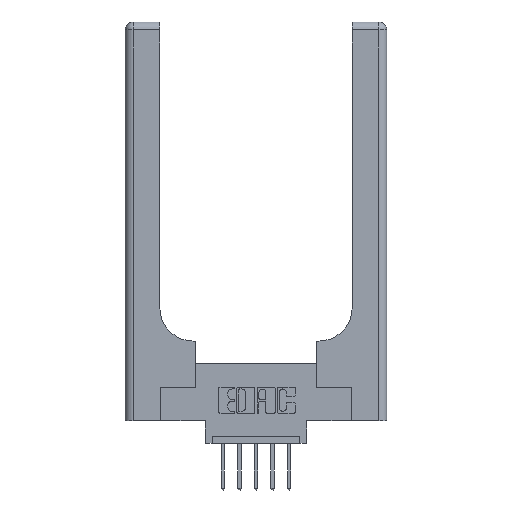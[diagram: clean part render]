
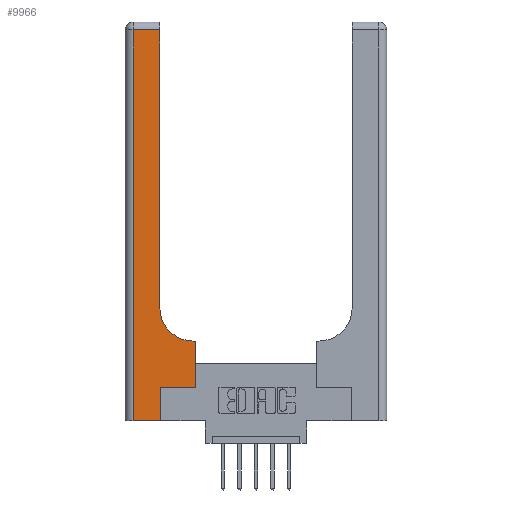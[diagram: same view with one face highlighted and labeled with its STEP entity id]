
A CAD part, top view. The second image highlights one B-rep face of the part: STEP entity #9966.
In plain terms, the highlighted planar face has unit normal (0, 0, 1).
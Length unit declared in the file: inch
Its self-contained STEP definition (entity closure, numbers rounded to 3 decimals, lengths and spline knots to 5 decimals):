
#115 = EDGE_CURVE ( 'NONE', #11340, #2435, #12974, .T. ) ;
#351 = EDGE_CURVE ( 'NONE', #13493, #11340, #6523, .T. ) ;
#663 = DIRECTION ( 'NONE',  ( 1., 0., 0. ) ) ;
#1074 = CARTESIAN_POINT ( 'NONE',  ( 0.26, 3., 0.37 ) ) ;
#1745 = ORIENTED_EDGE ( 'NONE', *, *, #12479, .T. ) ;
#1832 = VECTOR ( 'NONE', #2896, 39.37008 ) ;
#1881 = CARTESIAN_POINT ( 'NONE',  ( 0.265, 0., 0.37 ) ) ;
#1899 = CARTESIAN_POINT ( 'NONE',  ( 0.06, 0., 0.37 ) ) ;
#1978 = PLANE ( 'NONE',  #11228 ) ;
#1983 = VERTEX_POINT ( 'NONE', #2125 ) ;
#2125 = CARTESIAN_POINT ( 'NONE',  ( 0.265, 0.25, 0.37 ) ) ;
#2240 = LINE ( 'NONE', #9895, #9949 ) ;
#2265 = DIRECTION ( 'NONE',  ( 0., 1., 0. ) ) ;
#2435 = VERTEX_POINT ( 'NONE', #8600 ) ;
#2511 = LINE ( 'NONE', #13506, #4847 ) ;
#2845 = ORIENTED_EDGE ( 'NONE', *, *, #7144, .T. ) ;
#2877 = CARTESIAN_POINT ( 'NONE',  ( 0., 0., 0.37 ) ) ;
#2896 = DIRECTION ( 'NONE',  ( 1., 0., 0. ) ) ;
#2944 = DIRECTION ( 'NONE',  ( 1., 0., 0. ) ) ;
#3007 = CARTESIAN_POINT ( 'NONE',  ( 0.528, 0.25, 0.37 ) ) ;
#3360 = DIRECTION ( 'NONE',  ( -1., 0., 0. ) ) ;
#3731 = CARTESIAN_POINT ( 'NONE',  ( 0.51, 0.6, 0.37 ) ) ;
#3984 = ORIENTED_EDGE ( 'NONE', *, *, #6684, .T. ) ;
#4398 = CARTESIAN_POINT ( 'NONE',  ( 0.26, 0.6, 0.37 ) ) ;
#4427 = DIRECTION ( 'NONE',  ( 0., 1., 0. ) ) ;
#4812 = CARTESIAN_POINT ( 'NONE',  ( 0.528, 0.6, 0.37 ) ) ;
#4847 = VECTOR ( 'NONE', #4970, 39.37008 ) ;
#4906 = VERTEX_POINT ( 'NONE', #11835 ) ;
#4970 = DIRECTION ( 'NONE',  ( 0., -1., 0. ) ) ;
#5153 = CARTESIAN_POINT ( 'NONE',  ( 0.51, 0.85, 0.37 ) ) ;
#5369 = LINE ( 'NONE', #1074, #9426 ) ;
#5440 = DIRECTION ( 'NONE',  ( -1., 0., 0. ) ) ;
#5684 = EDGE_CURVE ( 'NONE', #6276, #6984, #13389, .T. ) ;
#5814 = VECTOR ( 'NONE', #11286, 39.37008 ) ;
#6146 = VECTOR ( 'NONE', #2944, 39.37008 ) ;
#6276 = VERTEX_POINT ( 'NONE', #1899 ) ;
#6316 = ORIENTED_EDGE ( 'NONE', *, *, #13641, .T. ) ;
#6484 = LINE ( 'NONE', #11822, #7961 ) ;
#6523 = LINE ( 'NONE', #4398, #5814 ) ;
#6579 = ORIENTED_EDGE ( 'NONE', *, *, #115, .T. ) ;
#6678 = ORIENTED_EDGE ( 'NONE', *, *, #351, .T. ) ;
#6684 = EDGE_CURVE ( 'NONE', #11587, #13493, #6484, .T. ) ;
#6935 = AXIS2_PLACEMENT_3D ( 'NONE', #5153, #9349, #663 ) ;
#6956 = EDGE_LOOP ( 'NONE', ( #2845, #6316, #10781, #9867, #1745, #12068, #3984, #6678, #6579 ) ) ;
#6984 = VERTEX_POINT ( 'NONE', #1881 ) ;
#7144 = EDGE_CURVE ( 'NONE', #2435, #9148, #5369, .T. ) ;
#7961 = VECTOR ( 'NONE', #9696, 39.37008 ) ;
#8245 = CARTESIAN_POINT ( 'NONE',  ( 0.265, 0.25, 0.37 ) ) ;
#8379 = VECTOR ( 'NONE', #4427, 39.37008 ) ;
#8480 = CARTESIAN_POINT ( 'NONE',  ( 0., 3., 0.37 ) ) ;
#8600 = CARTESIAN_POINT ( 'NONE',  ( 0.26, 0.85, 0.37 ) ) ;
#9148 = VERTEX_POINT ( 'NONE', #11177 ) ;
#9349 = DIRECTION ( 'NONE',  ( 0., 0., -1. ) ) ;
#9426 = VECTOR ( 'NONE', #2265, 39.37008 ) ;
#9635 = DIRECTION ( 'NONE',  ( 0., 0., -1. ) ) ;
#9696 = DIRECTION ( 'NONE',  ( 0., 1., 0. ) ) ;
#9759 = LINE ( 'NONE', #9820, #8379 ) ;
#9820 = CARTESIAN_POINT ( 'NONE',  ( 0.265, 0., 0.37 ) ) ;
#9867 = ORIENTED_EDGE ( 'NONE', *, *, #5684, .T. ) ;
#9895 = CARTESIAN_POINT ( 'NONE',  ( 0., 2.94, 0.37 ) ) ;
#9949 = VECTOR ( 'NONE', #3360, 39.37008 ) ;
#9966 = ADVANCED_FACE ( 'NONE', ( #13850 ), #1978, .F. ) ;
#10453 = EDGE_CURVE ( 'NONE', #4906, #6276, #2511, .T. ) ;
#10521 = LINE ( 'NONE', #8245, #1832 ) ;
#10781 = ORIENTED_EDGE ( 'NONE', *, *, #10453, .T. ) ;
#11177 = CARTESIAN_POINT ( 'NONE',  ( 0.26, 2.94, 0.37 ) ) ;
#11228 = AXIS2_PLACEMENT_3D ( 'NONE', #8480, #9635, #5440 ) ;
#11286 = DIRECTION ( 'NONE',  ( -1., 0., 0. ) ) ;
#11340 = VERTEX_POINT ( 'NONE', #3731 ) ;
#11587 = VERTEX_POINT ( 'NONE', #3007 ) ;
#11822 = CARTESIAN_POINT ( 'NONE',  ( 0.528, 0.25, 0.37 ) ) ;
#11835 = CARTESIAN_POINT ( 'NONE',  ( 0.06, 2.94, 0.37 ) ) ;
#12068 = ORIENTED_EDGE ( 'NONE', *, *, #12429, .T. ) ;
#12429 = EDGE_CURVE ( 'NONE', #1983, #11587, #10521, .T. ) ;
#12479 = EDGE_CURVE ( 'NONE', #6984, #1983, #9759, .T. ) ;
#12974 = CIRCLE ( 'NONE', #6935, 0.25 ) ;
#13389 = LINE ( 'NONE', #2877, #6146 ) ;
#13493 = VERTEX_POINT ( 'NONE', #4812 ) ;
#13506 = CARTESIAN_POINT ( 'NONE',  ( 0.06, 3., 0.37 ) ) ;
#13641 = EDGE_CURVE ( 'NONE', #9148, #4906, #2240, .T. ) ;
#13850 = FACE_OUTER_BOUND ( 'NONE', #6956, .T. ) ;
